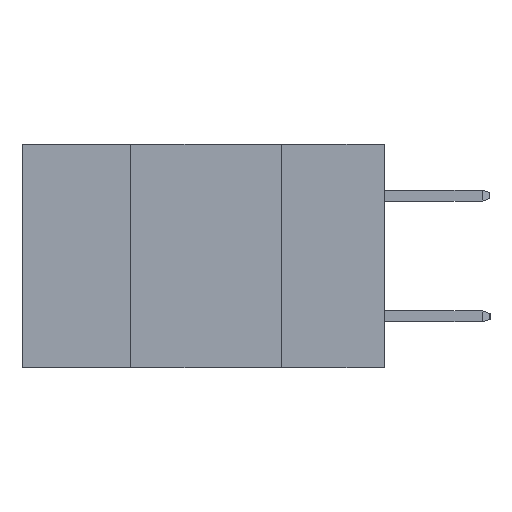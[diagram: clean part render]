
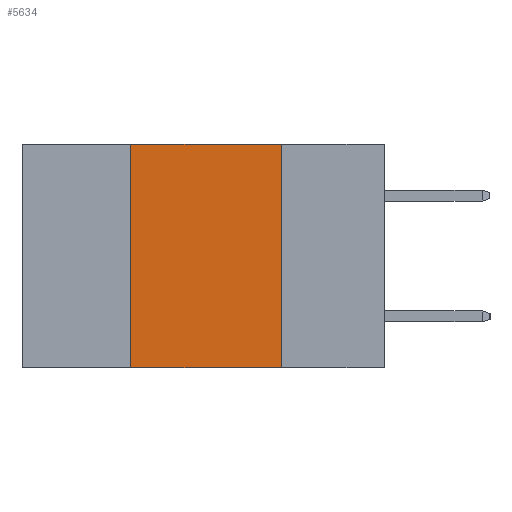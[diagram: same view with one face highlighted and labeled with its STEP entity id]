
A CAD part, left-side view. The second image highlights one B-rep face of the part: STEP entity #5634.
In plain terms, the highlighted planar face has unit normal (-1, 0, 0).
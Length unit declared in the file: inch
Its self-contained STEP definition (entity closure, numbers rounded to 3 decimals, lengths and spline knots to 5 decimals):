
#46 = VERTEX_POINT ( 'NONE', #9035 ) ;
#446 = LINE ( 'NONE', #12773, #2478 ) ;
#525 = AXIS2_PLACEMENT_3D ( 'NONE', #9655, #9641, #9627 ) ;
#539 = EDGE_LOOP ( 'NONE', ( #6102, #2947, #11182, #12508 ) ) ;
#1982 = LINE ( 'NONE', #7653, #6851 ) ;
#2478 = VECTOR ( 'NONE', #12748, 39.37008 ) ;
#2519 = CARTESIAN_POINT ( 'NONE',  ( 0., 0.42, -0.37 ) ) ;
#2947 = ORIENTED_EDGE ( 'NONE', *, *, #10264, .F. ) ;
#5447 = VECTOR ( 'NONE', #9780, 39.37008 ) ;
#5514 = VERTEX_POINT ( 'NONE', #10057 ) ;
#5634 = ADVANCED_FACE ( 'NONE', ( #11142 ), #9687, .F. ) ;
#5761 = LINE ( 'NONE', #10261, #5447 ) ;
#6102 = ORIENTED_EDGE ( 'NONE', *, *, #10419, .F. ) ;
#6851 = VECTOR ( 'NONE', #7347, 39.37008 ) ;
#7115 = VERTEX_POINT ( 'NONE', #2519 ) ;
#7347 = DIRECTION ( 'NONE',  ( 0., -1., 0. ) ) ;
#7653 = CARTESIAN_POINT ( 'NONE',  ( 0., 0.6, 0. ) ) ;
#7901 = VERTEX_POINT ( 'NONE', #8735 ) ;
#8735 = CARTESIAN_POINT ( 'NONE',  ( 0., 0.17, -0.37 ) ) ;
#9035 = CARTESIAN_POINT ( 'NONE',  ( 0., 0.42, 0. ) ) ;
#9627 = DIRECTION ( 'NONE',  ( 0., 0., -1. ) ) ;
#9641 = DIRECTION ( 'NONE',  ( 1., 0., 0. ) ) ;
#9655 = CARTESIAN_POINT ( 'NONE',  ( 0., 0.6, 0. ) ) ;
#9687 = PLANE ( 'NONE',  #525 ) ;
#9780 = DIRECTION ( 'NONE',  ( 0., 0., 1. ) ) ;
#10033 = LINE ( 'NONE', #12311, #12058 ) ;
#10057 = CARTESIAN_POINT ( 'NONE',  ( 0., 0.17, 0. ) ) ;
#10261 = CARTESIAN_POINT ( 'NONE',  ( 0., 0.42, -0.37 ) ) ;
#10264 = EDGE_CURVE ( 'NONE', #46, #5514, #1982, .T. ) ;
#10419 = EDGE_CURVE ( 'NONE', #5514, #7901, #446, .T. ) ;
#10465 = EDGE_CURVE ( 'NONE', #7115, #7901, #10033, .T. ) ;
#10590 = EDGE_CURVE ( 'NONE', #7115, #46, #5761, .T. ) ;
#11142 = FACE_OUTER_BOUND ( 'NONE', #539, .T. ) ;
#11182 = ORIENTED_EDGE ( 'NONE', *, *, #10590, .F. ) ;
#12058 = VECTOR ( 'NONE', #12264, 39.37008 ) ;
#12264 = DIRECTION ( 'NONE',  ( 0., -1., 0. ) ) ;
#12311 = CARTESIAN_POINT ( 'NONE',  ( 0., 0.6, -0.37 ) ) ;
#12508 = ORIENTED_EDGE ( 'NONE', *, *, #10465, .T. ) ;
#12748 = DIRECTION ( 'NONE',  ( 0., 0., -1. ) ) ;
#12773 = CARTESIAN_POINT ( 'NONE',  ( 0., 0.17, -0.37 ) ) ;
